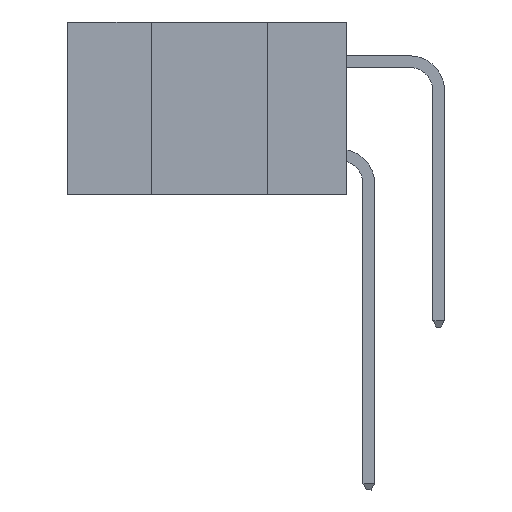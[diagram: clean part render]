
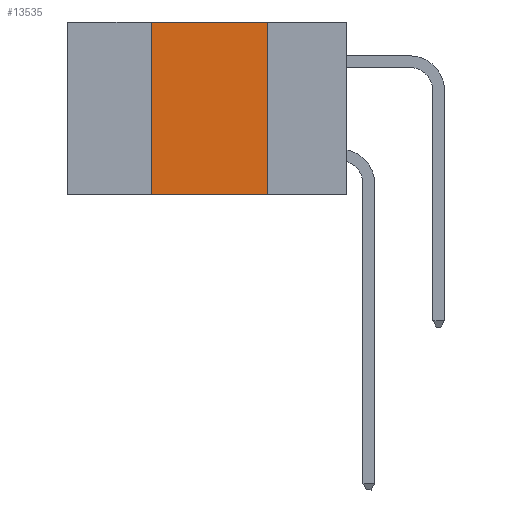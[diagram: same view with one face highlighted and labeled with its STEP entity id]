
A CAD part, left-side view. The second image highlights one B-rep face of the part: STEP entity #13535.
In plain terms, the highlighted planar face has unit normal (-1, 0, 0).
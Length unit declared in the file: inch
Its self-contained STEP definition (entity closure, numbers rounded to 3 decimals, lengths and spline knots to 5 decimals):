
#2321 = LINE ( 'NONE', #6979, #4520 ) ;
#2863 = CARTESIAN_POINT ( 'NONE',  ( 0., 0.17, 0. ) ) ;
#3615 = DIRECTION ( 'NONE',  ( 0., 0., 1. ) ) ;
#4477 = FACE_OUTER_BOUND ( 'NONE', #26929, .T. ) ;
#4520 = VECTOR ( 'NONE', #32710, 39.37008 ) ;
#5048 = VERTEX_POINT ( 'NONE', #29783 ) ;
#5499 = CARTESIAN_POINT ( 'NONE',  ( 0., 0.17, -0.37 ) ) ;
#5886 = VECTOR ( 'NONE', #46062, 39.37008 ) ;
#6979 = CARTESIAN_POINT ( 'NONE',  ( 0., 0.6, 0. ) ) ;
#7536 = CARTESIAN_POINT ( 'NONE',  ( 0., 0.6, 0. ) ) ;
#11921 = EDGE_CURVE ( 'NONE', #5048, #40349, #17468, .T. ) ;
#13081 = LINE ( 'NONE', #17281, #5886 ) ;
#13535 = ADVANCED_FACE ( 'NONE', ( #4477 ), #28846, .F. ) ;
#14101 = ORIENTED_EDGE ( 'NONE', *, *, #26950, .F. ) ;
#15968 = EDGE_CURVE ( 'NONE', #28016, #41298, #22999, .T. ) ;
#17202 = ORIENTED_EDGE ( 'NONE', *, *, #15968, .F. ) ;
#17281 = CARTESIAN_POINT ( 'NONE',  ( 0., 0.6, -0.37 ) ) ;
#17468 = LINE ( 'NONE', #46008, #30299 ) ;
#20506 = ORIENTED_EDGE ( 'NONE', *, *, #30292, .T. ) ;
#21835 = DIRECTION ( 'NONE',  ( 0., 0., -1. ) ) ;
#22999 = LINE ( 'NONE', #45660, #45923 ) ;
#25121 = DIRECTION ( 'NONE',  ( 1., 0., 0. ) ) ;
#26929 = EDGE_LOOP ( 'NONE', ( #17202, #14101, #28905, #20506 ) ) ;
#26950 = EDGE_CURVE ( 'NONE', #40349, #28016, #2321, .T. ) ;
#28016 = VERTEX_POINT ( 'NONE', #2863 ) ;
#28846 = PLANE ( 'NONE',  #38502 ) ;
#28905 = ORIENTED_EDGE ( 'NONE', *, *, #11921, .F. ) ;
#29783 = CARTESIAN_POINT ( 'NONE',  ( 0., 0.42, -0.37 ) ) ;
#30292 = EDGE_CURVE ( 'NONE', #5048, #41298, #13081, .T. ) ;
#30299 = VECTOR ( 'NONE', #3615, 39.37008 ) ;
#32710 = DIRECTION ( 'NONE',  ( 0., -1., 0. ) ) ;
#34384 = CARTESIAN_POINT ( 'NONE',  ( 0., 0.42, 0. ) ) ;
#38407 = DIRECTION ( 'NONE',  ( 0., 0., -1. ) ) ;
#38502 = AXIS2_PLACEMENT_3D ( 'NONE', #7536, #25121, #21835 ) ;
#40349 = VERTEX_POINT ( 'NONE', #34384 ) ;
#41298 = VERTEX_POINT ( 'NONE', #5499 ) ;
#45660 = CARTESIAN_POINT ( 'NONE',  ( 0., 0.17, 0. ) ) ;
#45923 = VECTOR ( 'NONE', #38407, 39.37008 ) ;
#46008 = CARTESIAN_POINT ( 'NONE',  ( 0., 0.42, 0. ) ) ;
#46062 = DIRECTION ( 'NONE',  ( 0., -1., 0. ) ) ;
